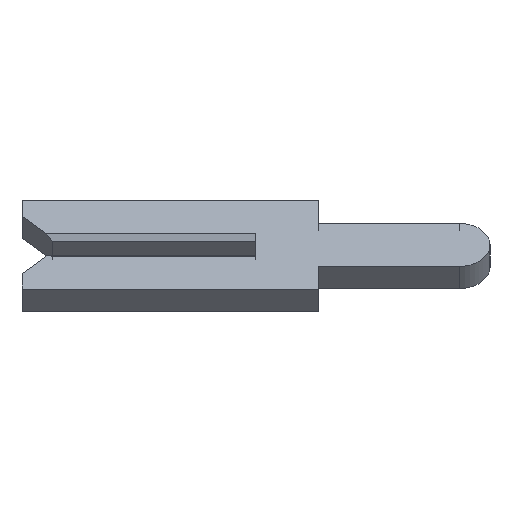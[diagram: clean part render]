
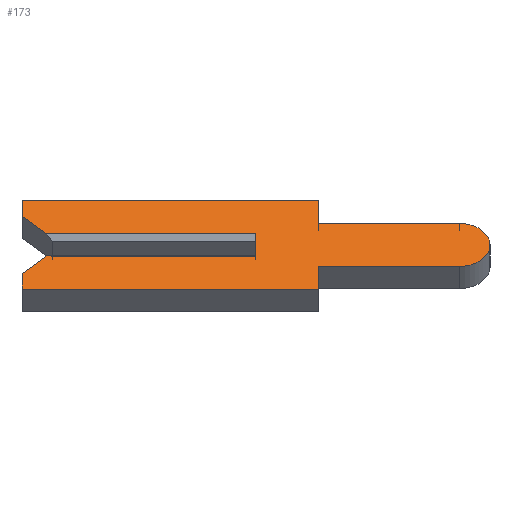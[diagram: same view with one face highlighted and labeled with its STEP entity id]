
A CAD part, left-side view. The second image highlights one B-rep face of the part: STEP entity #173.
In plain terms, the highlighted face is planar.
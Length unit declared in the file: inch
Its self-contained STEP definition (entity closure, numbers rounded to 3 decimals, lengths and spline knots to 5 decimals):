
#5 = VERTEX_POINT ( 'NONE', #374 ) ;
#7 = FACE_OUTER_BOUND ( 'NONE', #11, .T. ) ;
#11 = EDGE_LOOP ( 'NONE', ( #1271, #1008, #648, #553, #439, #583, #217, #905, #466, #517, #1427, #195, #310, #939 ) ) ;
#18 = LINE ( 'NONE', #1443, #20 ) ;
#19 = CARTESIAN_POINT ( 'NONE',  ( -0.01, -0.04, -0.0195 ) ) ;
#20 = VECTOR ( 'NONE', #549, 39.37008 ) ;
#40 = CARTESIAN_POINT ( 'NONE',  ( -0.01, 0., 0.01 ) ) ;
#56 = CARTESIAN_POINT ( 'NONE',  ( -0.01, 0.15, -0.026 ) ) ;
#71 = VERTEX_POINT ( 'NONE', #263 ) ;
#95 = DIRECTION ( 'NONE',  ( 0., -1., 0. ) ) ;
#118 = EDGE_CURVE ( 'NONE', #1575, #71, #1129, .T. ) ;
#127 = CARTESIAN_POINT ( 'NONE',  ( -0.01, -0.04, 0.0195 ) ) ;
#128 = AXIS2_PLACEMENT_3D ( 'NONE', #1319, #919, #162 ) ;
#162 = DIRECTION ( 'NONE',  ( 0., 0., -1. ) ) ;
#167 = DIRECTION ( 'NONE',  ( 0., -0.707, 0.707 ) ) ;
#171 = VECTOR ( 'NONE', #95, 39.37008 ) ;
#173 = ADVANCED_FACE ( 'NONE', ( #7 ), #688, .F. ) ;
#190 = DIRECTION ( 'NONE',  ( 0., 1., 0. ) ) ;
#195 = ORIENTED_EDGE ( 'NONE', *, *, #1112, .F. ) ;
#198 = CARTESIAN_POINT ( 'NONE',  ( -0.01, -0.04, 0.04 ) ) ;
#202 = VERTEX_POINT ( 'NONE', #40 ) ;
#213 = EDGE_CURVE ( 'NONE', #5, #202, #1247, .T. ) ;
#217 = ORIENTED_EDGE ( 'NONE', *, *, #1245, .F. ) ;
#229 = VERTEX_POINT ( 'NONE', #1193 ) ;
#238 = CIRCLE ( 'NONE', #1066, 0.0195 ) ;
#252 = DIRECTION ( 'NONE',  ( 0., -1., 0. ) ) ;
#263 = CARTESIAN_POINT ( 'NONE',  ( -0.01, 0., -0.01 ) ) ;
#276 = CARTESIAN_POINT ( 'NONE',  ( -0.01, 0.15, -0.026 ) ) ;
#283 = VERTEX_POINT ( 'NONE', #1303 ) ;
#310 = ORIENTED_EDGE ( 'NONE', *, *, #1383, .F. ) ;
#321 = DIRECTION ( 'NONE',  ( 0., 0., -1. ) ) ;
#338 = LINE ( 'NONE', #772, #1329 ) ;
#340 = CARTESIAN_POINT ( 'NONE',  ( -0.01, -0.1305, 0. ) ) ;
#374 = CARTESIAN_POINT ( 'NONE',  ( -0.01, 0.134, 0.01 ) ) ;
#405 = DIRECTION ( 'NONE',  ( 0., 0., 1. ) ) ;
#409 = EDGE_CURVE ( 'NONE', #811, #1546, #1399, .T. ) ;
#439 = ORIENTED_EDGE ( 'NONE', *, *, #409, .F. ) ;
#455 = CARTESIAN_POINT ( 'NONE',  ( -0.01, -0.04, -0.0195 ) ) ;
#461 = VECTOR ( 'NONE', #1027, 39.37008 ) ;
#466 = ORIENTED_EDGE ( 'NONE', *, *, #753, .F. ) ;
#493 = LINE ( 'NONE', #1544, #1489 ) ;
#495 = EDGE_CURVE ( 'NONE', #229, #811, #679, .T. ) ;
#503 = LINE ( 'NONE', #19, #593 ) ;
#517 = ORIENTED_EDGE ( 'NONE', *, *, #850, .F. ) ;
#549 = DIRECTION ( 'NONE',  ( 0., 0.707, 0.707 ) ) ;
#553 = ORIENTED_EDGE ( 'NONE', *, *, #1461, .F. ) ;
#557 = LINE ( 'NONE', #1587, #801 ) ;
#571 = VECTOR ( 'NONE', #190, 39.37008 ) ;
#583 = ORIENTED_EDGE ( 'NONE', *, *, #495, .F. ) ;
#593 = VECTOR ( 'NONE', #902, 39.37008 ) ;
#594 = DIRECTION ( 'NONE',  ( 0., 0., 1. ) ) ;
#597 = CARTESIAN_POINT ( 'NONE',  ( -0.01, 0., 0.0065 ) ) ;
#605 = VECTOR ( 'NONE', #594, 39.37008 ) ;
#648 = ORIENTED_EDGE ( 'NONE', *, *, #118, .F. ) ;
#652 = LINE ( 'NONE', #1564, #670 ) ;
#670 = VECTOR ( 'NONE', #167, 39.37008 ) ;
#679 = LINE ( 'NONE', #1611, #571 ) ;
#688 = PLANE ( 'NONE',  #128 ) ;
#712 = VERTEX_POINT ( 'NONE', #455 ) ;
#726 = EDGE_CURVE ( 'NONE', #1168, #1201, #1278, .T. ) ;
#733 = DIRECTION ( 'NONE',  ( 0., 0., -1. ) ) ;
#753 = EDGE_CURVE ( 'NONE', #283, #840, #238, .T. ) ;
#763 = CARTESIAN_POINT ( 'NONE',  ( -0.01, -0.1305, -0.01 ) ) ;
#766 = CARTESIAN_POINT ( 'NONE',  ( -0.01, -0.04, 0.04 ) ) ;
#772 = CARTESIAN_POINT ( 'NONE',  ( -0.01, 0.15, 0.04 ) ) ;
#801 = VECTOR ( 'NONE', #808, 39.37008 ) ;
#804 = DIRECTION ( 'NONE',  ( 0., -1., 0. ) ) ;
#808 = DIRECTION ( 'NONE',  ( 0., 0., 1. ) ) ;
#811 = VERTEX_POINT ( 'NONE', #1241 ) ;
#820 = EDGE_CURVE ( 'NONE', #71, #202, #1284, .T. ) ;
#840 = VERTEX_POINT ( 'NONE', #1368 ) ;
#850 = EDGE_CURVE ( 'NONE', #1201, #283, #869, .T. ) ;
#853 = DIRECTION ( 'NONE',  ( 1., 0., 0. ) ) ;
#869 = LINE ( 'NONE', #1501, #171 ) ;
#902 = DIRECTION ( 'NONE',  ( 0., 1., 0. ) ) ;
#905 = ORIENTED_EDGE ( 'NONE', *, *, #1210, .F. ) ;
#919 = DIRECTION ( 'NONE',  ( 1., 0., 0. ) ) ;
#924 = CARTESIAN_POINT ( 'NONE',  ( -0.01, 0.15, 0.01 ) ) ;
#939 = ORIENTED_EDGE ( 'NONE', *, *, #1334, .F. ) ;
#943 = VECTOR ( 'NONE', #804, 39.37008 ) ;
#1008 = ORIENTED_EDGE ( 'NONE', *, *, #820, .F. ) ;
#1027 = DIRECTION ( 'NONE',  ( 0., -1., 0. ) ) ;
#1039 = VERTEX_POINT ( 'NONE', #1617 ) ;
#1044 = VECTOR ( 'NONE', #405, 39.37008 ) ;
#1066 = AXIS2_PLACEMENT_3D ( 'NONE', #340, #853, #733 ) ;
#1112 = EDGE_CURVE ( 'NONE', #1466, #1168, #338, .T. ) ;
#1129 = LINE ( 'NONE', #763, #461 ) ;
#1164 = CARTESIAN_POINT ( 'NONE',  ( -0.01, 0.15, 0.04 ) ) ;
#1168 = VERTEX_POINT ( 'NONE', #766 ) ;
#1193 = CARTESIAN_POINT ( 'NONE',  ( -0.01, -0.04, -0.04 ) ) ;
#1201 = VERTEX_POINT ( 'NONE', #127 ) ;
#1210 = EDGE_CURVE ( 'NONE', #840, #712, #503, .T. ) ;
#1241 = CARTESIAN_POINT ( 'NONE',  ( -0.01, 0.15, -0.04 ) ) ;
#1245 = EDGE_CURVE ( 'NONE', #712, #229, #493, .T. ) ;
#1247 = LINE ( 'NONE', #924, #943 ) ;
#1271 = ORIENTED_EDGE ( 'NONE', *, *, #213, .T. ) ;
#1278 = LINE ( 'NONE', #198, #1512 ) ;
#1284 = LINE ( 'NONE', #597, #605 ) ;
#1287 = DIRECTION ( 'NONE',  ( 0., 0., -1. ) ) ;
#1303 = CARTESIAN_POINT ( 'NONE',  ( -0.01, -0.1305, 0.0195 ) ) ;
#1310 = CARTESIAN_POINT ( 'NONE',  ( -0.01, 0.134, -0.01 ) ) ;
#1319 = CARTESIAN_POINT ( 'NONE',  ( -0.01, -0.1305, 0. ) ) ;
#1329 = VECTOR ( 'NONE', #252, 39.37008 ) ;
#1334 = EDGE_CURVE ( 'NONE', #5, #1039, #18, .T. ) ;
#1368 = CARTESIAN_POINT ( 'NONE',  ( -0.01, -0.1305, -0.0195 ) ) ;
#1383 = EDGE_CURVE ( 'NONE', #1039, #1466, #557, .T. ) ;
#1399 = LINE ( 'NONE', #276, #1044 ) ;
#1427 = ORIENTED_EDGE ( 'NONE', *, *, #726, .F. ) ;
#1443 = CARTESIAN_POINT ( 'NONE',  ( -0.01, 0.1305, 0.0065 ) ) ;
#1461 = EDGE_CURVE ( 'NONE', #1546, #1575, #652, .T. ) ;
#1466 = VERTEX_POINT ( 'NONE', #1164 ) ;
#1489 = VECTOR ( 'NONE', #1287, 39.37008 ) ;
#1501 = CARTESIAN_POINT ( 'NONE',  ( -0.01, -0.04, 0.0195 ) ) ;
#1512 = VECTOR ( 'NONE', #321, 39.37008 ) ;
#1544 = CARTESIAN_POINT ( 'NONE',  ( -0.01, -0.04, -0.04 ) ) ;
#1546 = VERTEX_POINT ( 'NONE', #56 ) ;
#1564 = CARTESIAN_POINT ( 'NONE',  ( -0.01, 0.1305, -0.0065 ) ) ;
#1575 = VERTEX_POINT ( 'NONE', #1310 ) ;
#1587 = CARTESIAN_POINT ( 'NONE',  ( -0.01, 0.15, 0.026 ) ) ;
#1611 = CARTESIAN_POINT ( 'NONE',  ( -0.01, 0.15, -0.04 ) ) ;
#1617 = CARTESIAN_POINT ( 'NONE',  ( -0.01, 0.15, 0.026 ) ) ;
